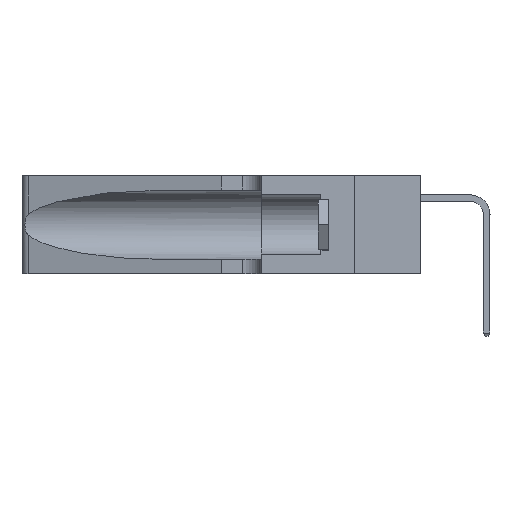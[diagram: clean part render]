
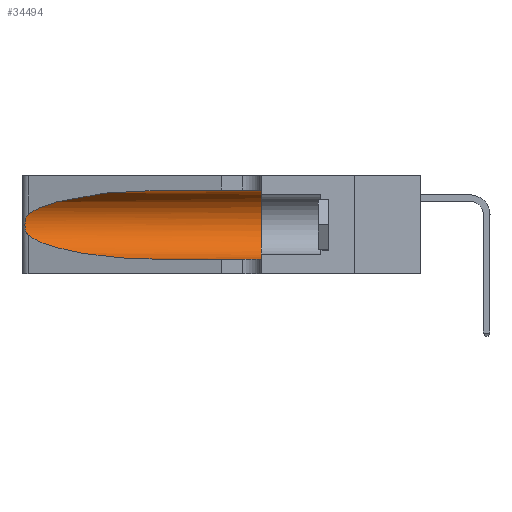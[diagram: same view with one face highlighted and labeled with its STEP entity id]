
A CAD part, left-side view. The second image highlights one B-rep face of the part: STEP entity #34494.
In plain terms, the highlighted cylindrical face has radius 3.308 mm (diameter 6.617 mm), a partial arc.
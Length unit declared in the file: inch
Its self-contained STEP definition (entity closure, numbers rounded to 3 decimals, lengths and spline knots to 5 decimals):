
#59 = CIRCLE ( 'NONE', #40699, 0.13025 ) ;
#226 = CYLINDRICAL_SURFACE ( 'NONE', #37773, 0.13025 ) ;
#455 = CARTESIAN_POINT ( 'NONE',  ( 0.25787, 1.23484, 0.2124 ) ) ;
#1756 = VERTEX_POINT ( 'NONE', #12861 ) ;
#2463 = CARTESIAN_POINT ( 'NONE',  ( 0.25487, 1.22718, 0.22369 ) ) ;
#2511 = CARTESIAN_POINT ( 'NONE',  ( 0.2373, 1.15595, 0.08982 ) ) ;
#2802 = VECTOR ( 'NONE', #12097, 39.37008 ) ;
#3697 = CARTESIAN_POINT ( 'NONE',  ( 0.26018, 1.23835, 0.19895 ) ) ;
#4362 = EDGE_LOOP ( 'NONE', ( #26204, #39300, #23316, #13670, #34605, #28842 ) ) ;
#4682 = CARTESIAN_POINT ( 'NONE',  ( 0.1305, 0.72297, 0.31525 ) ) ;
#5892 = CARTESIAN_POINT ( 'NONE',  ( 0.1305, 1.61858, 0.05475 ) ) ;
#6261 = EDGE_CURVE ( 'NONE', #30918, #39677, #59, .T. ) ;
#6941 = CARTESIAN_POINT ( 'NONE',  ( 0.26075, 1.23896, 0.178 ) ) ;
#7609 = EDGE_CURVE ( 'NONE', #20161, #11705, #11366, .T. ) ;
#7764 =( BOUNDED_CURVE ( )  B_SPLINE_CURVE ( 3, ( #20268, #33080, #33222, #13892 ),
 .UNSPECIFIED., .F., .T. ) 
 B_SPLINE_CURVE_WITH_KNOTS ( ( 4, 4 ),
 ( 1.5708, 2.84003 ),
 .UNSPECIFIED. ) 
 CURVE ( )  GEOMETRIC_REPRESENTATION_ITEM ( )  RATIONAL_B_SPLINE_CURVE ( ( 1., 0.87, 0.87, 1. ) ) 
 REPRESENTATION_ITEM ( '' )  );
#10175 = CARTESIAN_POINT ( 'NONE',  ( 0.25856, 1.23593, 0.16098 ) ) ;
#11366 = B_SPLINE_CURVE_WITH_KNOTS ( 'NONE', 3,
 ( #39200, #16647, #35926, #455, #23098, #3697, #26337, #6941, #29576, #10175, #32836, #13483, #36064, #16785 ),
 .UNSPECIFIED., .F., .F.,
 ( 4, 2, 2, 2, 2, 2, 4 ),
 ( 0., 0.00027, 0.00053, 0.00107, 0.0016, 0.00187, 0.00214 ),
 .UNSPECIFIED. ) ;
#11705 = VERTEX_POINT ( 'NONE', #34154 ) ;
#11840 = EDGE_CURVE ( 'NONE', #29673, #30918, #19033, .T. ) ;
#12097 = DIRECTION ( 'NONE',  ( 0., -1., 0. ) ) ;
#12256 = CARTESIAN_POINT ( 'NONE',  ( 0.18966, 0.96281, 0.05475 ) ) ;
#12861 = CARTESIAN_POINT ( 'NONE',  ( 0.1305, 0.72297, 0.05475 ) ) ;
#13483 = CARTESIAN_POINT ( 'NONE',  ( 0.25639, 1.23186, 0.15144 ) ) ;
#13670 = ORIENTED_EDGE ( 'NONE', *, *, #28577, .T. ) ;
#13892 = CARTESIAN_POINT ( 'NONE',  ( 0.25487, 1.22718, 0.22369 ) ) ;
#14960 = LINE ( 'NONE', #5892, #40719 ) ;
#15097 = DIRECTION ( 'NONE',  ( 0., 1., 0. ) ) ;
#16647 = CARTESIAN_POINT ( 'NONE',  ( 0.25555, 1.22994, 0.2215 ) ) ;
#16670 =( BOUNDED_CURVE ( )  B_SPLINE_CURVE ( 3, ( #25151, #2511, #12256, #34869 ),
 .UNSPECIFIED., .F., .F. ) 
 B_SPLINE_CURVE_WITH_KNOTS ( ( 4, 4 ),
 ( 3.44316, 4.71239 ),
 .UNSPECIFIED. ) 
 CURVE ( )  GEOMETRIC_REPRESENTATION_ITEM ( )  RATIONAL_B_SPLINE_CURVE ( ( 1., 0.87, 0.87, 1. ) ) 
 REPRESENTATION_ITEM ( '' )  );
#16785 = CARTESIAN_POINT ( 'NONE',  ( 0.25487, 1.22718, 0.14631 ) ) ;
#18093 = EDGE_CURVE ( 'NONE', #11705, #1756, #16670, .T. ) ;
#18616 = CARTESIAN_POINT ( 'NONE',  ( 0.1305, 1.61858, 0.185 ) ) ;
#19033 = LINE ( 'NONE', #37966, #2802 ) ;
#19512 = FACE_OUTER_BOUND ( 'NONE', #4362, .T. ) ;
#20161 = VERTEX_POINT ( 'NONE', #2463 ) ;
#20268 = CARTESIAN_POINT ( 'NONE',  ( 0.1305, 0.72297, 0.31525 ) ) ;
#21845 = DIRECTION ( 'NONE',  ( 0., -1., 0. ) ) ;
#23098 = CARTESIAN_POINT ( 'NONE',  ( 0.25854, 1.2359, 0.20912 ) ) ;
#23316 = ORIENTED_EDGE ( 'NONE', *, *, #18093, .T. ) ;
#23869 = CARTESIAN_POINT ( 'NONE',  ( 0.1305, 0.35, 0.05475 ) ) ;
#25151 = CARTESIAN_POINT ( 'NONE',  ( 0.25487, 1.22718, 0.14631 ) ) ;
#26204 = ORIENTED_EDGE ( 'NONE', *, *, #28221, .T. ) ;
#26337 = CARTESIAN_POINT ( 'NONE',  ( 0.26075, 1.23896, 0.19203 ) ) ;
#26925 = CARTESIAN_POINT ( 'NONE',  ( 0.1305, 0.35, 0.31525 ) ) ;
#28221 = EDGE_CURVE ( 'NONE', #29673, #20161, #7764, .T. ) ;
#28577 = EDGE_CURVE ( 'NONE', #1756, #39677, #14960, .T. ) ;
#28842 = ORIENTED_EDGE ( 'NONE', *, *, #11840, .F. ) ;
#29576 = CARTESIAN_POINT ( 'NONE',  ( 0.26017, 1.23833, 0.17102 ) ) ;
#29673 = VERTEX_POINT ( 'NONE', #4682 ) ;
#30918 = VERTEX_POINT ( 'NONE', #26925 ) ;
#31423 = DIRECTION ( 'NONE',  ( 0., 0., -1. ) ) ;
#31779 = DIRECTION ( 'NONE',  ( 0., -1., 0. ) ) ;
#32836 = CARTESIAN_POINT ( 'NONE',  ( 0.25789, 1.23486, 0.15765 ) ) ;
#33080 = CARTESIAN_POINT ( 'NONE',  ( 0.18966, 0.96281, 0.31525 ) ) ;
#33222 = CARTESIAN_POINT ( 'NONE',  ( 0.2373, 1.15595, 0.28018 ) ) ;
#34154 = CARTESIAN_POINT ( 'NONE',  ( 0.25487, 1.22718, 0.14631 ) ) ;
#34406 = CARTESIAN_POINT ( 'NONE',  ( 0.1305, 0.35, 0.185 ) ) ;
#34494 = ADVANCED_FACE ( 'NONE', ( #19512 ), #226, .F. ) ;
#34605 = ORIENTED_EDGE ( 'NONE', *, *, #6261, .F. ) ;
#34869 = CARTESIAN_POINT ( 'NONE',  ( 0.1305, 0.72297, 0.05475 ) ) ;
#35926 = CARTESIAN_POINT ( 'NONE',  ( 0.25639, 1.23184, 0.21858 ) ) ;
#36064 = CARTESIAN_POINT ( 'NONE',  ( 0.25555, 1.22993, 0.14849 ) ) ;
#37680 = DIRECTION ( 'NONE',  ( 0., 0., 1. ) ) ;
#37773 = AXIS2_PLACEMENT_3D ( 'NONE', #18616, #21845, #31423 ) ;
#37966 = CARTESIAN_POINT ( 'NONE',  ( 0.1305, 1.61858, 0.31525 ) ) ;
#39200 = CARTESIAN_POINT ( 'NONE',  ( 0.25487, 1.22718, 0.22369 ) ) ;
#39300 = ORIENTED_EDGE ( 'NONE', *, *, #7609, .T. ) ;
#39677 = VERTEX_POINT ( 'NONE', #23869 ) ;
#40699 = AXIS2_PLACEMENT_3D ( 'NONE', #34406, #15097, #37680 ) ;
#40719 = VECTOR ( 'NONE', #31779, 39.37008 ) ;
